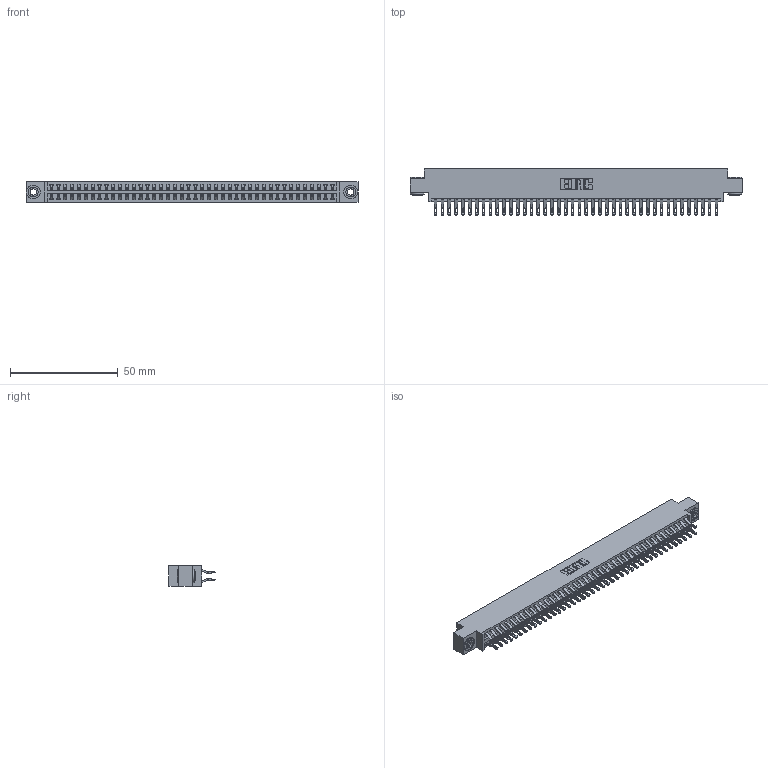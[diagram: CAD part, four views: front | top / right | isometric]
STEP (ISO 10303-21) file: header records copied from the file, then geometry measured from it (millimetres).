
FILE_DESCRIPTION (( 'STEP AP203' ), '1' );
FILE_NAME ('346-084-555-803.STEP', '2022-05-25T20:30:37', ( '' ), ( '' ), 'SwSTEP 2.0', 'SolidWorks 2020', '' );
FILE_SCHEMA (( 'CONFIG_CONTROL_DESIGN' ));
Length unit declared in the file: inch
Products named in the file (4): 346-084-555-803; 345-292-001_555 Tail; 345-250-002_345-250-002-102; 346 Part_0.170 Offset - 0.156 Dia-TH
Assembly tree (87 placements, depth 2):
  346-084-555-803
    346 Part_0.170 Offset - 0.156 Dia-TH
    345-292-001_555 Tail  x84
    345-250-002_345-250-002-102  x2
Bounding box: 153.92 x 21.46 x 9.4 mm (x, y, z)
Volume: 15099.8 mm3; surface area: 22052.6 mm2
Topology: 87 solids, 87 shells, 5050 faces, 15825 edges, 10546 vertices
Faces by surface type: plane 2876, cylinder 2166, cone 8
Entity records: 28934 total; most frequent: CARTESIAN_POINT 4787, ORIENTED_EDGE 4682, DIRECTION 4267, EDGE_CURVE 2341, LINE 1997, VECTOR 1997, VERTEX_POINT 1558, AXIS2_PLACEMENT_3D 1135
